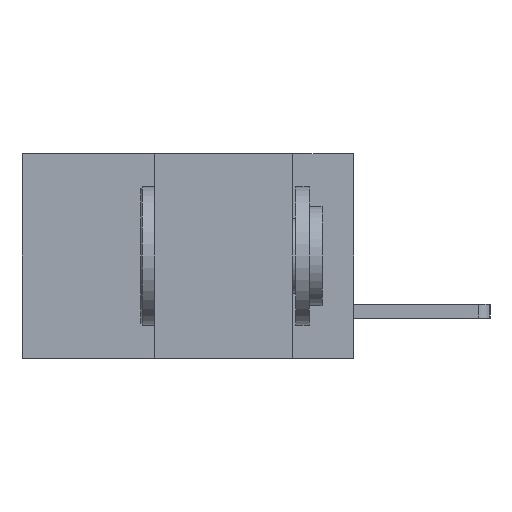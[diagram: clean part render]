
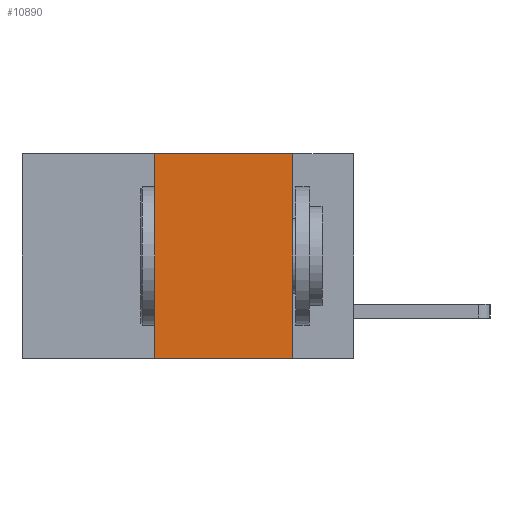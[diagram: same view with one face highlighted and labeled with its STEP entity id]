
A CAD part, left-side view. The second image highlights one B-rep face of the part: STEP entity #10890.
In plain terms, the highlighted planar face has unit normal (-1, 0, 0).
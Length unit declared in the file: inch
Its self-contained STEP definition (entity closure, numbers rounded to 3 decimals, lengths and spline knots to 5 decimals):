
#7 = CARTESIAN_POINT ( 'NONE',  ( 0., 0.6, 0. ) ) ;
#235 = CARTESIAN_POINT ( 'NONE',  ( 0., 0.36, 0. ) ) ;
#539 = CARTESIAN_POINT ( 'NONE',  ( 0., 0.36, -0.37 ) ) ;
#589 = LINE ( 'NONE', #7945, #10886 ) ;
#1159 = CARTESIAN_POINT ( 'NONE',  ( 0., 0.11, 0. ) ) ;
#1234 = DIRECTION ( 'NONE',  ( 1., 0., 0. ) ) ;
#1425 = CARTESIAN_POINT ( 'NONE',  ( 0., 0.11, 0. ) ) ;
#1632 = VECTOR ( 'NONE', #10071, 39.37008 ) ;
#2133 = ORIENTED_EDGE ( 'NONE', *, *, #4300, .F. ) ;
#2554 = CARTESIAN_POINT ( 'NONE',  ( 0., 0.11, -0.37 ) ) ;
#2612 = VERTEX_POINT ( 'NONE', #2554 ) ;
#2645 = EDGE_CURVE ( 'NONE', #4018, #2612, #589, .T. ) ;
#3642 = CARTESIAN_POINT ( 'NONE',  ( 0., 0.36, 0. ) ) ;
#4018 = VERTEX_POINT ( 'NONE', #539 ) ;
#4300 = EDGE_CURVE ( 'NONE', #4018, #9539, #10139, .T. ) ;
#4491 = CARTESIAN_POINT ( 'NONE',  ( 0., 0.6, 0. ) ) ;
#4559 = AXIS2_PLACEMENT_3D ( 'NONE', #4491, #1234, #4563 ) ;
#4563 = DIRECTION ( 'NONE',  ( 0., 0., -1. ) ) ;
#5477 = ORIENTED_EDGE ( 'NONE', *, *, #6217, .F. ) ;
#5672 = PLANE ( 'NONE',  #4559 ) ;
#5798 = EDGE_LOOP ( 'NONE', ( #8150, #5477, #2133, #11641 ) ) ;
#6082 = DIRECTION ( 'NONE',  ( 0., -1., 0. ) ) ;
#6217 = EDGE_CURVE ( 'NONE', #9539, #12579, #9540, .T. ) ;
#6296 = LINE ( 'NONE', #1159, #13243 ) ;
#7472 = DIRECTION ( 'NONE',  ( 0., -1., 0. ) ) ;
#7945 = CARTESIAN_POINT ( 'NONE',  ( 0., 0.6, -0.37 ) ) ;
#8150 = ORIENTED_EDGE ( 'NONE', *, *, #10805, .F. ) ;
#9539 = VERTEX_POINT ( 'NONE', #235 ) ;
#9540 = LINE ( 'NONE', #7, #12104 ) ;
#10071 = DIRECTION ( 'NONE',  ( 0., 0., 1. ) ) ;
#10139 = LINE ( 'NONE', #3642, #1632 ) ;
#10666 = DIRECTION ( 'NONE',  ( 0., 0., -1. ) ) ;
#10805 = EDGE_CURVE ( 'NONE', #12579, #2612, #6296, .T. ) ;
#10886 = VECTOR ( 'NONE', #6082, 39.37008 ) ;
#10890 = ADVANCED_FACE ( 'NONE', ( #12924 ), #5672, .F. ) ;
#11641 = ORIENTED_EDGE ( 'NONE', *, *, #2645, .T. ) ;
#12104 = VECTOR ( 'NONE', #7472, 39.37008 ) ;
#12579 = VERTEX_POINT ( 'NONE', #1425 ) ;
#12924 = FACE_OUTER_BOUND ( 'NONE', #5798, .T. ) ;
#13243 = VECTOR ( 'NONE', #10666, 39.37008 ) ;
